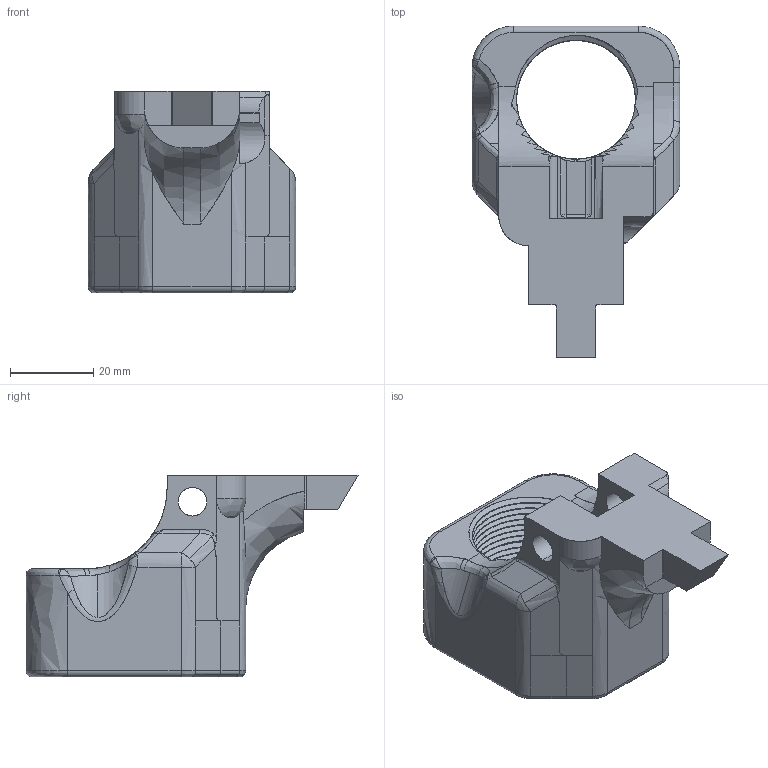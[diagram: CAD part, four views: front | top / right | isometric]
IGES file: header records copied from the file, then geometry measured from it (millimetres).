
Start section: SolidWorks IGES file using analytic representation for surfaces
Global section: file name: Hermes_V1.4_Rear.IGS; native system: SolidWorks 2015; preprocessor: SolidWorks 2015; author: WarFairy; date: 150521.101215; units: inch
Bounding box: 50 x 79.86 x 48.55 mm (x, y, z)
Surface area: 17499.7 mm2 (no closed solid volume)
Topology: 0 solids, 0 shells, 223 faces, 2917 edges, 2912 vertices
Faces by surface type: bspline 117, revolution 106
